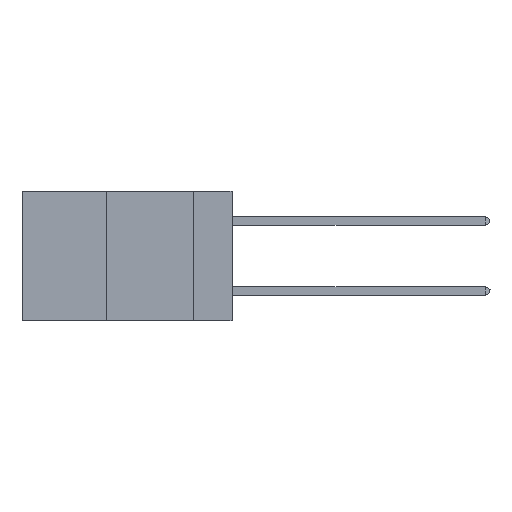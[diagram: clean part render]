
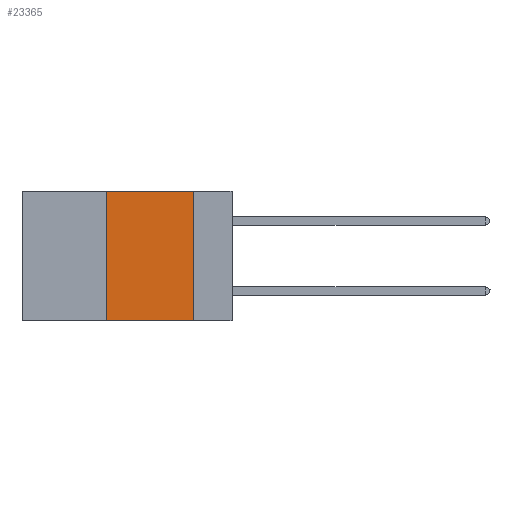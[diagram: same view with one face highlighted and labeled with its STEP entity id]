
A CAD part, left-side view. The second image highlights one B-rep face of the part: STEP entity #23365.
In plain terms, the highlighted planar face has unit normal (-1, 0, 0).
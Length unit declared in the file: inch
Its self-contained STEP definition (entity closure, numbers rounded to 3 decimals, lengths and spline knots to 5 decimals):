
#912 = VECTOR ( 'NONE', #12754, 39.37008 ) ;
#1333 = VECTOR ( 'NONE', #17371, 39.37008 ) ;
#3001 = CARTESIAN_POINT ( 'NONE',  ( 0., 0.6, 0. ) ) ;
#4230 = ORIENTED_EDGE ( 'NONE', *, *, #39569, .T. ) ;
#4938 = DIRECTION ( 'NONE',  ( 1., 0., 0. ) ) ;
#4967 = CARTESIAN_POINT ( 'NONE',  ( 0., 0.11, -0.37 ) ) ;
#5105 = ORIENTED_EDGE ( 'NONE', *, *, #38474, .F. ) ;
#6386 = LINE ( 'NONE', #21064, #1333 ) ;
#7300 = DIRECTION ( 'NONE',  ( 0., 0., -1. ) ) ;
#7363 = CARTESIAN_POINT ( 'NONE',  ( 0., 0.11, 0. ) ) ;
#7752 = CARTESIAN_POINT ( 'NONE',  ( 0., 0.6, 0. ) ) ;
#8287 = CARTESIAN_POINT ( 'NONE',  ( 0., 0.36, 0. ) ) ;
#11108 = DIRECTION ( 'NONE',  ( 0., 0., -1. ) ) ;
#11925 = VECTOR ( 'NONE', #7300, 39.37008 ) ;
#12537 = LINE ( 'NONE', #3001, #912 ) ;
#12754 = DIRECTION ( 'NONE',  ( 0., -1., 0. ) ) ;
#14213 = EDGE_LOOP ( 'NONE', ( #27086, #5105, #39065, #4230 ) ) ;
#14381 = LINE ( 'NONE', #8287, #20510 ) ;
#16750 = VERTEX_POINT ( 'NONE', #4967 ) ;
#17371 = DIRECTION ( 'NONE',  ( 0., -1., 0. ) ) ;
#17728 = EDGE_CURVE ( 'NONE', #31073, #16750, #18562, .T. ) ;
#18119 = FACE_OUTER_BOUND ( 'NONE', #14213, .T. ) ;
#18562 = LINE ( 'NONE', #36959, #11925 ) ;
#19731 = CARTESIAN_POINT ( 'NONE',  ( 0., 0.36, -0.37 ) ) ;
#20231 = EDGE_CURVE ( 'NONE', #38487, #26450, #14381, .T. ) ;
#20510 = VECTOR ( 'NONE', #37266, 39.37008 ) ;
#21064 = CARTESIAN_POINT ( 'NONE',  ( 0., 0.6, -0.37 ) ) ;
#23365 = ADVANCED_FACE ( 'NONE', ( #18119 ), #27220, .F. ) ;
#26450 = VERTEX_POINT ( 'NONE', #30242 ) ;
#26718 = AXIS2_PLACEMENT_3D ( 'NONE', #7752, #4938, #11108 ) ;
#27086 = ORIENTED_EDGE ( 'NONE', *, *, #17728, .F. ) ;
#27220 = PLANE ( 'NONE',  #26718 ) ;
#30242 = CARTESIAN_POINT ( 'NONE',  ( 0., 0.36, 0. ) ) ;
#31073 = VERTEX_POINT ( 'NONE', #7363 ) ;
#36959 = CARTESIAN_POINT ( 'NONE',  ( 0., 0.11, 0. ) ) ;
#37266 = DIRECTION ( 'NONE',  ( 0., 0., 1. ) ) ;
#38474 = EDGE_CURVE ( 'NONE', #26450, #31073, #12537, .T. ) ;
#38487 = VERTEX_POINT ( 'NONE', #19731 ) ;
#39065 = ORIENTED_EDGE ( 'NONE', *, *, #20231, .F. ) ;
#39569 = EDGE_CURVE ( 'NONE', #38487, #16750, #6386, .T. ) ;
